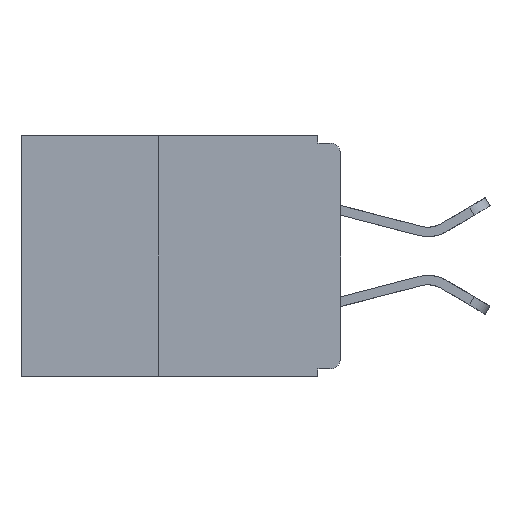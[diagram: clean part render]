
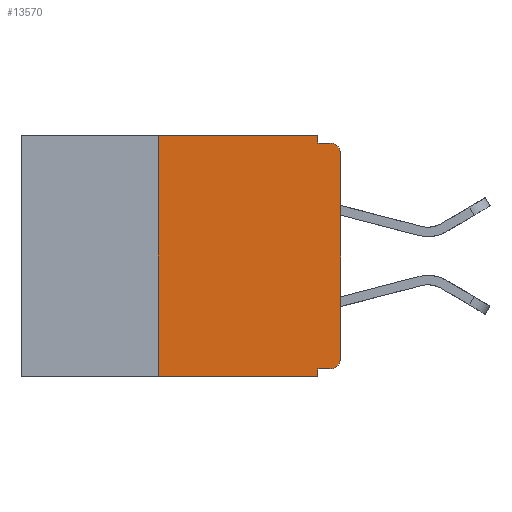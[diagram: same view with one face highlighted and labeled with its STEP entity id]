
A CAD part, left-side view. The second image highlights one B-rep face of the part: STEP entity #13570.
In plain terms, the highlighted planar face has unit normal (-1, 0, 0).
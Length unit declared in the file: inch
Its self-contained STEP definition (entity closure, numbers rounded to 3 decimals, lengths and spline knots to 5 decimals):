
#148 = CIRCLE ( 'NONE', #6462, 0.015 ) ;
#299 = ORIENTED_EDGE ( 'NONE', *, *, #22062, .T. ) ;
#330 = ORIENTED_EDGE ( 'NONE', *, *, #6923, .T. ) ;
#895 = VERTEX_POINT ( 'NONE', #24334 ) ;
#1038 = LINE ( 'NONE', #6626, #15190 ) ;
#1233 = ORIENTED_EDGE ( 'NONE', *, *, #27631, .F. ) ;
#1454 = ORIENTED_EDGE ( 'NONE', *, *, #4998, .F. ) ;
#1819 = ORIENTED_EDGE ( 'NONE', *, *, #27290, .F. ) ;
#1880 = ORIENTED_EDGE ( 'NONE', *, *, #23457, .F. ) ;
#2218 = ORIENTED_EDGE ( 'NONE', *, *, #26404, .T. ) ;
#2299 = VERTEX_POINT ( 'NONE', #6320 ) ;
#2882 = ORIENTED_EDGE ( 'NONE', *, *, #34046, .F. ) ;
#2977 = EDGE_CURVE ( 'NONE', #10230, #895, #1038, .T. ) ;
#3361 = ORIENTED_EDGE ( 'NONE', *, *, #2977, .F. ) ;
#3401 = VECTOR ( 'NONE', #15322, 39.37008 ) ;
#3428 = ORIENTED_EDGE ( 'NONE', *, *, #12378, .T. ) ;
#4234 = FACE_OUTER_BOUND ( 'NONE', #33578, .T. ) ;
#4329 = VECTOR ( 'NONE', #32657, 39.37008 ) ;
#4343 = LINE ( 'NONE', #28491, #31640 ) ;
#4998 = EDGE_CURVE ( 'NONE', #22296, #22606, #9180, .T. ) ;
#5033 = VERTEX_POINT ( 'NONE', #28232 ) ;
#5107 = CARTESIAN_POINT ( 'NONE',  ( 0., 0.031, -0.01 ) ) ;
#6197 = CARTESIAN_POINT ( 'NONE',  ( 0., 0.437, -0.33 ) ) ;
#6320 = CARTESIAN_POINT ( 'NONE',  ( 0., 0.031, -0.33 ) ) ;
#6462 = AXIS2_PLACEMENT_3D ( 'NONE', #11827, #30335, #14510 ) ;
#6465 = VERTEX_POINT ( 'NONE', #31637 ) ;
#6626 = CARTESIAN_POINT ( 'NONE',  ( 0., 0., -0.32 ) ) ;
#6711 = LINE ( 'NONE', #8764, #12931 ) ;
#6923 = EDGE_CURVE ( 'NONE', #5033, #6465, #19467, .T. ) ;
#7916 = AXIS2_PLACEMENT_3D ( 'NONE', #15583, #33940, #18237 ) ;
#8231 = CARTESIAN_POINT ( 'NONE',  ( 0., 0.25, -0.33 ) ) ;
#8397 = PLANE ( 'NONE',  #32826 ) ;
#8764 = CARTESIAN_POINT ( 'NONE',  ( 0., 0., -0.01 ) ) ;
#9180 = LINE ( 'NONE', #12226, #21659 ) ;
#9513 = VERTEX_POINT ( 'NONE', #8231 ) ;
#9912 = DIRECTION ( 'NONE',  ( 0., 0., -1. ) ) ;
#10170 = VECTOR ( 'NONE', #21745, 39.37008 ) ;
#10230 = VERTEX_POINT ( 'NONE', #11086 ) ;
#10944 = CARTESIAN_POINT ( 'NONE',  ( 0., 0.437, 0. ) ) ;
#11086 = CARTESIAN_POINT ( 'NONE',  ( 0., 0.015, -0.32 ) ) ;
#11827 = CARTESIAN_POINT ( 'NONE',  ( 0., 0.015, -0.305 ) ) ;
#12226 = CARTESIAN_POINT ( 'NONE',  ( 0., 0.031, 0. ) ) ;
#12378 = EDGE_CURVE ( 'NONE', #10230, #21644, #148, .T. ) ;
#12642 = CARTESIAN_POINT ( 'NONE',  ( 0., 0.437, 0. ) ) ;
#12931 = VECTOR ( 'NONE', #14121, 39.37008 ) ;
#13570 = ADVANCED_FACE ( 'NONE', ( #4234 ), #8397, .F. ) ;
#14121 = DIRECTION ( 'NONE',  ( 0., -1., 0. ) ) ;
#14510 = DIRECTION ( 'NONE',  ( 0., 0., -1. ) ) ;
#15190 = VECTOR ( 'NONE', #27862, 39.37008 ) ;
#15322 = DIRECTION ( 'NONE',  ( 0., -1., 0. ) ) ;
#15583 = CARTESIAN_POINT ( 'NONE',  ( 0., 0.015, -0.025 ) ) ;
#16412 = DIRECTION ( 'NONE',  ( 0., 0., -1. ) ) ;
#17446 = DIRECTION ( 'NONE',  ( 0., 0., -1. ) ) ;
#18237 = DIRECTION ( 'NONE',  ( 0., 0., -1. ) ) ;
#18419 = LINE ( 'NONE', #6197, #4329 ) ;
#18793 = CARTESIAN_POINT ( 'NONE',  ( 0., 0., -0.305 ) ) ;
#19067 = CARTESIAN_POINT ( 'NONE',  ( 0., 0.25, -0.33 ) ) ;
#19467 = CIRCLE ( 'NONE', #7916, 0.015 ) ;
#21644 = VERTEX_POINT ( 'NONE', #18793 ) ;
#21659 = VECTOR ( 'NONE', #17446, 39.37008 ) ;
#21745 = DIRECTION ( 'NONE',  ( 0., 0., 1. ) ) ;
#22062 = EDGE_CURVE ( 'NONE', #21644, #5033, #32996, .T. ) ;
#22296 = VERTEX_POINT ( 'NONE', #24946 ) ;
#22606 = VERTEX_POINT ( 'NONE', #5107 ) ;
#23185 = CARTESIAN_POINT ( 'NONE',  ( 0., 0.25, 0. ) ) ;
#23457 = EDGE_CURVE ( 'NONE', #9513, #31797, #31283, .T. ) ;
#24334 = CARTESIAN_POINT ( 'NONE',  ( 0., 0.031, -0.32 ) ) ;
#24566 = LINE ( 'NONE', #12642, #3401 ) ;
#24946 = CARTESIAN_POINT ( 'NONE',  ( 0., 0.031, 0. ) ) ;
#26404 = EDGE_CURVE ( 'NONE', #9513, #2299, #18419, .T. ) ;
#26884 = VECTOR ( 'NONE', #30892, 39.37008 ) ;
#27290 = EDGE_CURVE ( 'NONE', #31797, #22296, #24566, .T. ) ;
#27631 = EDGE_CURVE ( 'NONE', #22606, #6465, #6711, .T. ) ;
#27862 = DIRECTION ( 'NONE',  ( 0., 1., 0. ) ) ;
#28232 = CARTESIAN_POINT ( 'NONE',  ( 0., 0., -0.025 ) ) ;
#28491 = CARTESIAN_POINT ( 'NONE',  ( 0., 0.031, -0.33 ) ) ;
#30335 = DIRECTION ( 'NONE',  ( -1., 0., 0. ) ) ;
#30892 = DIRECTION ( 'NONE',  ( 0., 0., 1. ) ) ;
#31283 = LINE ( 'NONE', #19067, #10170 ) ;
#31637 = CARTESIAN_POINT ( 'NONE',  ( 0., 0.015, -0.01 ) ) ;
#31640 = VECTOR ( 'NONE', #9912, 39.37008 ) ;
#31797 = VERTEX_POINT ( 'NONE', #23185 ) ;
#32202 = DIRECTION ( 'NONE',  ( 1., 0., 0. ) ) ;
#32657 = DIRECTION ( 'NONE',  ( 0., -1., 0. ) ) ;
#32826 = AXIS2_PLACEMENT_3D ( 'NONE', #10944, #32202, #16412 ) ;
#32996 = LINE ( 'NONE', #33682, #26884 ) ;
#33578 = EDGE_LOOP ( 'NONE', ( #299, #330, #1233, #1454, #1819, #1880, #2218, #2882, #3361, #3428 ) ) ;
#33682 = CARTESIAN_POINT ( 'NONE',  ( 0., 0., 0. ) ) ;
#33940 = DIRECTION ( 'NONE',  ( -1., 0., 0. ) ) ;
#34046 = EDGE_CURVE ( 'NONE', #895, #2299, #4343, .T. ) ;
